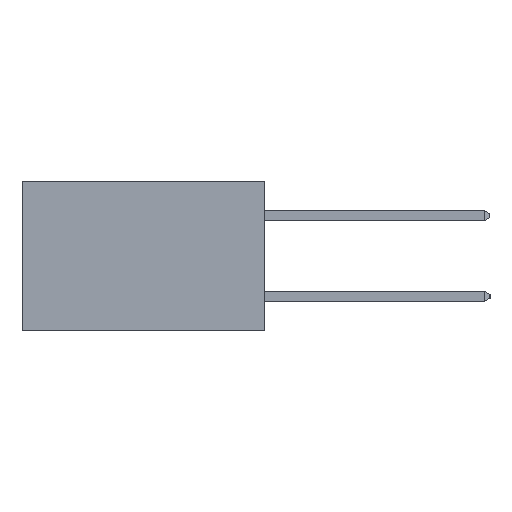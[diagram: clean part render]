
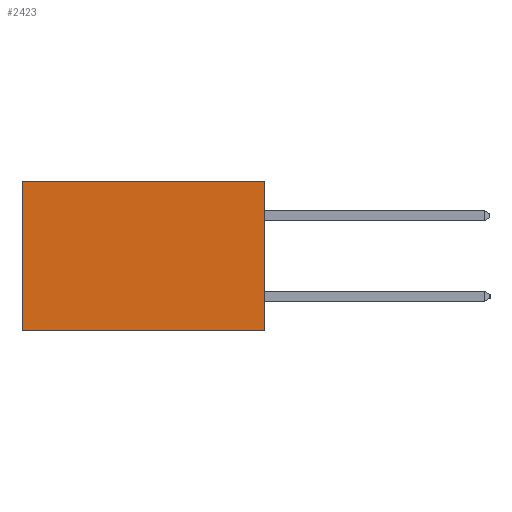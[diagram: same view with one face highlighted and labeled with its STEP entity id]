
A CAD part, left-side view. The second image highlights one B-rep face of the part: STEP entity #2423.
In plain terms, the highlighted planar face has unit normal (-1, 0, 0).
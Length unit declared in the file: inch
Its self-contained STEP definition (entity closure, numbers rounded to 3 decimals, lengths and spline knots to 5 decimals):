
#448 = EDGE_LOOP ( 'NONE', ( #7519, #4231, #8617, #12783 ) ) ;
#1242 = EDGE_CURVE ( 'NONE', #10074, #16238, #7799, .T. ) ;
#2423 = ADVANCED_FACE ( 'NONE', ( #9399 ), #5836, .F. ) ;
#2997 = CARTESIAN_POINT ( 'NONE',  ( 0.2615, 0., -0.37 ) ) ;
#3667 = CARTESIAN_POINT ( 'NONE',  ( 0.2615, 0., 0. ) ) ;
#3788 = LINE ( 'NONE', #9821, #13874 ) ;
#4042 = DIRECTION ( 'NONE',  ( 0., 0., -1. ) ) ;
#4231 = ORIENTED_EDGE ( 'NONE', *, *, #4684, .F. ) ;
#4485 = CARTESIAN_POINT ( 'NONE',  ( 0.2615, 0., -0.37 ) ) ;
#4684 = EDGE_CURVE ( 'NONE', #16238, #5607, #6476, .T. ) ;
#5607 = VERTEX_POINT ( 'NONE', #6189 ) ;
#5678 = DIRECTION ( 'NONE',  ( 0., 0., -1. ) ) ;
#5698 = DIRECTION ( 'NONE',  ( 1., 0., 0. ) ) ;
#5720 = CARTESIAN_POINT ( 'NONE',  ( 0.2615, 0., -0.37 ) ) ;
#5836 = PLANE ( 'NONE',  #14334 ) ;
#6003 = EDGE_CURVE ( 'NONE', #10074, #11742, #11145, .T. ) ;
#6057 = CARTESIAN_POINT ( 'NONE',  ( 0.2615, 0., -0.37 ) ) ;
#6189 = CARTESIAN_POINT ( 'NONE',  ( 0.2615, 0.6, -0.37 ) ) ;
#6476 = LINE ( 'NONE', #2997, #13017 ) ;
#7519 = ORIENTED_EDGE ( 'NONE', *, *, #15456, .T. ) ;
#7799 = LINE ( 'NONE', #4485, #10478 ) ;
#8617 = ORIENTED_EDGE ( 'NONE', *, *, #1242, .F. ) ;
#9399 = FACE_OUTER_BOUND ( 'NONE', #448, .T. ) ;
#9821 = CARTESIAN_POINT ( 'NONE',  ( 0.2615, 0.6, -0.37 ) ) ;
#9869 = CARTESIAN_POINT ( 'NONE',  ( 0.2615, 0.6, 0. ) ) ;
#10074 = VERTEX_POINT ( 'NONE', #3667 ) ;
#10478 = VECTOR ( 'NONE', #4042, 39.37008 ) ;
#11145 = LINE ( 'NONE', #15792, #11555 ) ;
#11555 = VECTOR ( 'NONE', #15650, 39.37008 ) ;
#11742 = VERTEX_POINT ( 'NONE', #9869 ) ;
#12783 = ORIENTED_EDGE ( 'NONE', *, *, #6003, .T. ) ;
#13017 = VECTOR ( 'NONE', #16453, 39.37008 ) ;
#13874 = VECTOR ( 'NONE', #16229, 39.37008 ) ;
#14334 = AXIS2_PLACEMENT_3D ( 'NONE', #5720, #5698, #5678 ) ;
#15456 = EDGE_CURVE ( 'NONE', #11742, #5607, #3788, .T. ) ;
#15650 = DIRECTION ( 'NONE',  ( 0., 1., 0. ) ) ;
#15792 = CARTESIAN_POINT ( 'NONE',  ( 0.2615, 0., 0. ) ) ;
#16229 = DIRECTION ( 'NONE',  ( 0., 0., -1. ) ) ;
#16238 = VERTEX_POINT ( 'NONE', #6057 ) ;
#16453 = DIRECTION ( 'NONE',  ( 0., 1., 0. ) ) ;
